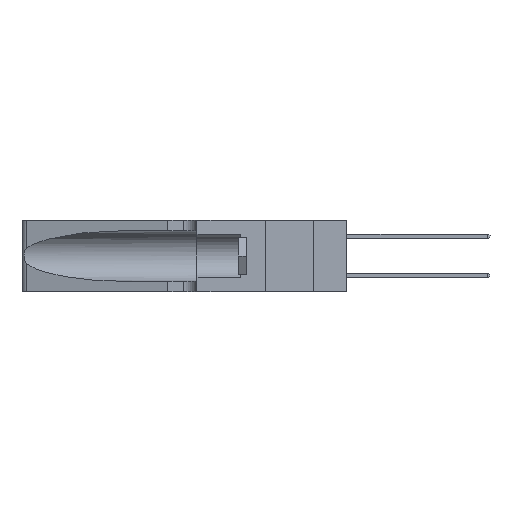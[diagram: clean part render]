
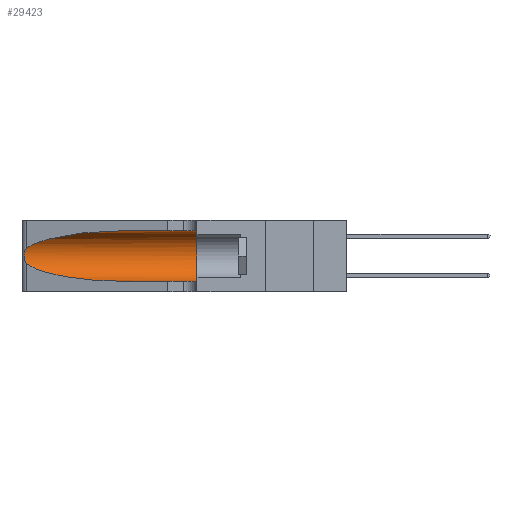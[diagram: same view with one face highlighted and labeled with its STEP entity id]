
A CAD part, left-side view. The second image highlights one B-rep face of the part: STEP entity #29423.
In plain terms, the highlighted cylindrical face has radius 3.308 mm (diameter 6.617 mm), a partial arc.
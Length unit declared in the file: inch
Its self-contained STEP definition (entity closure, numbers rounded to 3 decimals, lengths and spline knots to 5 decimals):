
#40 = LINE ( 'NONE', #668, #24401 ) ;
#151 = CIRCLE ( 'NONE', #11495, 0.13025 ) ;
#168 = DIRECTION ( 'NONE',  ( 0., -1., 0. ) ) ;
#668 = CARTESIAN_POINT ( 'NONE',  ( 0.1305, 1.61858, 0.05475 ) ) ;
#1878 = CARTESIAN_POINT ( 'NONE',  ( 0.25639, 1.23184, 0.21858 ) ) ;
#2161 = ORIENTED_EDGE ( 'NONE', *, *, #13282, .T. ) ;
#2572 = CARTESIAN_POINT ( 'NONE',  ( 0.25789, 1.23486, 0.15765 ) ) ;
#2655 = CARTESIAN_POINT ( 'NONE',  ( 0.25487, 1.22718, 0.14631 ) ) ;
#3472 = B_SPLINE_CURVE_WITH_KNOTS ( 'NONE', 3,
 ( #31960, #16474, #1878, #19728, #12290, #27157, #15738, #5669, #26270, #27068, #2572, #20842, #14834, #2655 ),
 .UNSPECIFIED., .F., .F.,
 ( 4, 2, 2, 2, 2, 2, 4 ),
 ( 0., 0.00027, 0.00053, 0.00107, 0.0016, 0.00187, 0.00214 ),
 .UNSPECIFIED. ) ;
#4289 = CARTESIAN_POINT ( 'NONE',  ( 0.1305, 0.35, 0.185 ) ) ;
#5669 = CARTESIAN_POINT ( 'NONE',  ( 0.26075, 1.23896, 0.178 ) ) ;
#6883 = EDGE_CURVE ( 'NONE', #30570, #17552, #23766, .T. ) ;
#6891 = VECTOR ( 'NONE', #27168, 39.37008 ) ;
#7958 = CYLINDRICAL_SURFACE ( 'NONE', #11903, 0.13025 ) ;
#8858 = ORIENTED_EDGE ( 'NONE', *, *, #6883, .T. ) ;
#11440 = EDGE_CURVE ( 'NONE', #27901, #11852, #151, .T. ) ;
#11474 = ORIENTED_EDGE ( 'NONE', *, *, #28383, .T. ) ;
#11495 = AXIS2_PLACEMENT_3D ( 'NONE', #4289, #32137, #19324 ) ;
#11852 = VERTEX_POINT ( 'NONE', #24346 ) ;
#11903 = AXIS2_PLACEMENT_3D ( 'NONE', #33103, #168, #17732 ) ;
#12290 = CARTESIAN_POINT ( 'NONE',  ( 0.25854, 1.2359, 0.20912 ) ) ;
#13282 = EDGE_CURVE ( 'NONE', #28964, #30570, #3472, .T. ) ;
#13532 = CARTESIAN_POINT ( 'NONE',  ( 0.2373, 1.15595, 0.28018 ) ) ;
#13757 = DIRECTION ( 'NONE',  ( 0., -1., 0. ) ) ;
#14029 = CARTESIAN_POINT ( 'NONE',  ( 0.1305, 0.35, 0.31525 ) ) ;
#14335 = FACE_OUTER_BOUND ( 'NONE', #26906, .T. ) ;
#14834 = CARTESIAN_POINT ( 'NONE',  ( 0.25555, 1.22993, 0.14849 ) ) ;
#15738 = CARTESIAN_POINT ( 'NONE',  ( 0.26075, 1.23896, 0.19203 ) ) ;
#16365 = CARTESIAN_POINT ( 'NONE',  ( 0.1305, 0.72297, 0.05475 ) ) ;
#16474 = CARTESIAN_POINT ( 'NONE',  ( 0.25555, 1.22994, 0.2215 ) ) ;
#17552 = VERTEX_POINT ( 'NONE', #16365 ) ;
#17560 = CARTESIAN_POINT ( 'NONE',  ( 0.1305, 0.72297, 0.31525 ) ) ;
#17732 = DIRECTION ( 'NONE',  ( 0., 0., -1. ) ) ;
#18020 = EDGE_CURVE ( 'NONE', #27628, #28964, #25824, .T. ) ;
#18742 = CARTESIAN_POINT ( 'NONE',  ( 0.25487, 1.22718, 0.14631 ) ) ;
#19324 = DIRECTION ( 'NONE',  ( 0., 0., 1. ) ) ;
#19728 = CARTESIAN_POINT ( 'NONE',  ( 0.25787, 1.23484, 0.2124 ) ) ;
#20704 = CARTESIAN_POINT ( 'NONE',  ( 0.1305, 0.72297, 0.31525 ) ) ;
#20842 = CARTESIAN_POINT ( 'NONE',  ( 0.25639, 1.23186, 0.15144 ) ) ;
#21126 = CARTESIAN_POINT ( 'NONE',  ( 0.18966, 0.96281, 0.31525 ) ) ;
#21299 = CARTESIAN_POINT ( 'NONE',  ( 0.18966, 0.96281, 0.05475 ) ) ;
#22086 = CARTESIAN_POINT ( 'NONE',  ( 0.25487, 1.22718, 0.14631 ) ) ;
#23155 = ORIENTED_EDGE ( 'NONE', *, *, #11440, .F. ) ;
#23300 = EDGE_CURVE ( 'NONE', #27628, #27901, #23673, .T. ) ;
#23673 = LINE ( 'NONE', #29487, #6891 ) ;
#23766 =( BOUNDED_CURVE ( )  B_SPLINE_CURVE ( 3, ( #18742, #26253, #21299, #29039 ),
 .UNSPECIFIED., .F., .F. ) 
 B_SPLINE_CURVE_WITH_KNOTS ( ( 4, 4 ),
 ( 3.44316, 4.71239 ),
 .UNSPECIFIED. ) 
 CURVE ( )  GEOMETRIC_REPRESENTATION_ITEM ( )  RATIONAL_B_SPLINE_CURVE ( ( 1., 0.87, 0.87, 1. ) ) 
 REPRESENTATION_ITEM ( '' )  );
#24346 = CARTESIAN_POINT ( 'NONE',  ( 0.1305, 0.35, 0.05475 ) ) ;
#24401 = VECTOR ( 'NONE', #13757, 39.37008 ) ;
#25824 =( BOUNDED_CURVE ( )  B_SPLINE_CURVE ( 3, ( #20704, #21126, #13532, #31459 ),
 .UNSPECIFIED., .F., .F. ) 
 B_SPLINE_CURVE_WITH_KNOTS ( ( 4, 4 ),
 ( 1.5708, 2.84003 ),
 .UNSPECIFIED. ) 
 CURVE ( )  GEOMETRIC_REPRESENTATION_ITEM ( )  RATIONAL_B_SPLINE_CURVE ( ( 1., 0.87, 0.87, 1. ) ) 
 REPRESENTATION_ITEM ( '' )  );
#26253 = CARTESIAN_POINT ( 'NONE',  ( 0.2373, 1.15595, 0.08982 ) ) ;
#26270 = CARTESIAN_POINT ( 'NONE',  ( 0.26017, 1.23833, 0.17102 ) ) ;
#26549 = CARTESIAN_POINT ( 'NONE',  ( 0.25487, 1.22718, 0.22369 ) ) ;
#26635 = ORIENTED_EDGE ( 'NONE', *, *, #18020, .T. ) ;
#26906 = EDGE_LOOP ( 'NONE', ( #26635, #2161, #8858, #11474, #23155, #29265 ) ) ;
#27068 = CARTESIAN_POINT ( 'NONE',  ( 0.25856, 1.23593, 0.16098 ) ) ;
#27157 = CARTESIAN_POINT ( 'NONE',  ( 0.26018, 1.23835, 0.19895 ) ) ;
#27168 = DIRECTION ( 'NONE',  ( 0., -1., 0. ) ) ;
#27628 = VERTEX_POINT ( 'NONE', #17560 ) ;
#27901 = VERTEX_POINT ( 'NONE', #14029 ) ;
#28383 = EDGE_CURVE ( 'NONE', #17552, #11852, #40, .T. ) ;
#28964 = VERTEX_POINT ( 'NONE', #26549 ) ;
#29039 = CARTESIAN_POINT ( 'NONE',  ( 0.1305, 0.72297, 0.05475 ) ) ;
#29265 = ORIENTED_EDGE ( 'NONE', *, *, #23300, .F. ) ;
#29423 = ADVANCED_FACE ( 'NONE', ( #14335 ), #7958, .F. ) ;
#29487 = CARTESIAN_POINT ( 'NONE',  ( 0.1305, 1.61858, 0.31525 ) ) ;
#30570 = VERTEX_POINT ( 'NONE', #22086 ) ;
#31459 = CARTESIAN_POINT ( 'NONE',  ( 0.25487, 1.22718, 0.22369 ) ) ;
#31960 = CARTESIAN_POINT ( 'NONE',  ( 0.25487, 1.22718, 0.22369 ) ) ;
#32137 = DIRECTION ( 'NONE',  ( 0., 1., 0. ) ) ;
#33103 = CARTESIAN_POINT ( 'NONE',  ( 0.1305, 1.61858, 0.185 ) ) ;
